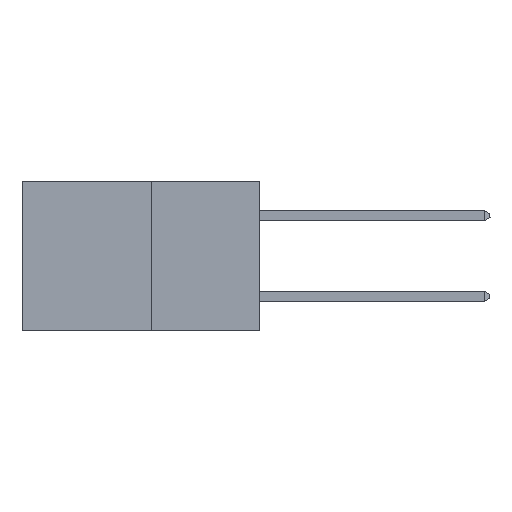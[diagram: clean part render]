
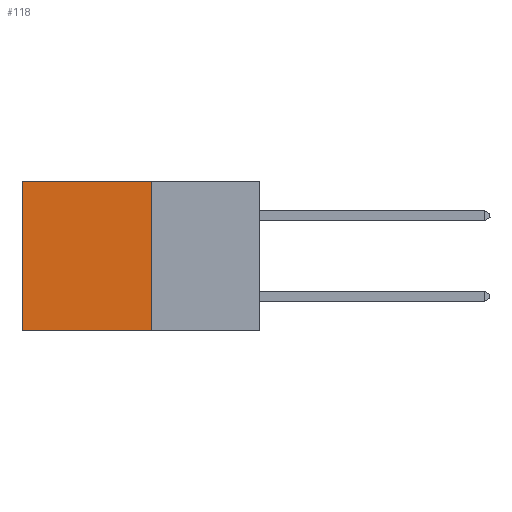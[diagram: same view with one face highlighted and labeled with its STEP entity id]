
A CAD part, left-side view. The second image highlights one B-rep face of the part: STEP entity #118.
In plain terms, the highlighted planar face has unit normal (-1, 0, 0).
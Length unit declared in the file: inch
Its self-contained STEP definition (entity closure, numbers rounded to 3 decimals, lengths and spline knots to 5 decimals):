
#118 = ADVANCED_FACE ( 'NONE', ( #27645 ), #32714, .F. ) ;
#1331 = EDGE_LOOP ( 'NONE', ( #7634, #17516, #7417, #13958 ) ) ;
#3762 = CARTESIAN_POINT ( 'NONE',  ( 0.277, 0.59, -0.37 ) ) ;
#5050 = DIRECTION ( 'NONE',  ( 0., 0., -1. ) ) ;
#5144 = VERTEX_POINT ( 'NONE', #13388 ) ;
#5269 = LINE ( 'NONE', #31850, #25851 ) ;
#5473 = EDGE_CURVE ( 'NONE', #33934, #20503, #13869, .T. ) ;
#7417 = ORIENTED_EDGE ( 'NONE', *, *, #7809, .F. ) ;
#7506 = VECTOR ( 'NONE', #15236, 39.37008 ) ;
#7634 = ORIENTED_EDGE ( 'NONE', *, *, #27882, .T. ) ;
#7809 = EDGE_CURVE ( 'NONE', #33934, #12850, #5269, .T. ) ;
#8357 = LINE ( 'NONE', #23696, #9212 ) ;
#9212 = VECTOR ( 'NONE', #26398, 39.37008 ) ;
#11821 = CARTESIAN_POINT ( 'NONE',  ( 0.277, 0.27, -0.37 ) ) ;
#12379 = VECTOR ( 'NONE', #30673, 39.37008 ) ;
#12850 = VERTEX_POINT ( 'NONE', #33994 ) ;
#13388 = CARTESIAN_POINT ( 'NONE',  ( 0.277, 0.59, -0.37 ) ) ;
#13869 = LINE ( 'NONE', #31291, #7506 ) ;
#13958 = ORIENTED_EDGE ( 'NONE', *, *, #5473, .T. ) ;
#15236 = DIRECTION ( 'NONE',  ( 0., 1., 0. ) ) ;
#15755 = CARTESIAN_POINT ( 'NONE',  ( 0.277, 0.27, 0. ) ) ;
#17516 = ORIENTED_EDGE ( 'NONE', *, *, #21392, .F. ) ;
#19472 = LINE ( 'NONE', #3762, #12379 ) ;
#20004 = CARTESIAN_POINT ( 'NONE',  ( 0.277, 0.59, 0. ) ) ;
#20503 = VERTEX_POINT ( 'NONE', #20004 ) ;
#21392 = EDGE_CURVE ( 'NONE', #12850, #5144, #8357, .T. ) ;
#22127 = DIRECTION ( 'NONE',  ( 0., 0., -1. ) ) ;
#22419 = DIRECTION ( 'NONE',  ( 1., 0., 0. ) ) ;
#23696 = CARTESIAN_POINT ( 'NONE',  ( 0.277, 0.27, -0.37 ) ) ;
#25851 = VECTOR ( 'NONE', #5050, 39.37008 ) ;
#26398 = DIRECTION ( 'NONE',  ( 0., 1., 0. ) ) ;
#27230 = AXIS2_PLACEMENT_3D ( 'NONE', #11821, #22419, #22127 ) ;
#27645 = FACE_OUTER_BOUND ( 'NONE', #1331, .T. ) ;
#27882 = EDGE_CURVE ( 'NONE', #20503, #5144, #19472, .T. ) ;
#30673 = DIRECTION ( 'NONE',  ( 0., 0., -1. ) ) ;
#31291 = CARTESIAN_POINT ( 'NONE',  ( 0.277, 0.27, 0. ) ) ;
#31850 = CARTESIAN_POINT ( 'NONE',  ( 0.277, 0.27, -0.37 ) ) ;
#32714 = PLANE ( 'NONE',  #27230 ) ;
#33934 = VERTEX_POINT ( 'NONE', #15755 ) ;
#33994 = CARTESIAN_POINT ( 'NONE',  ( 0.277, 0.27, -0.37 ) ) ;
